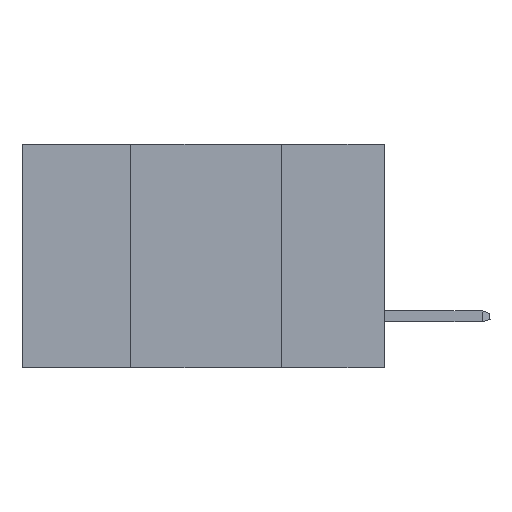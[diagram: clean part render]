
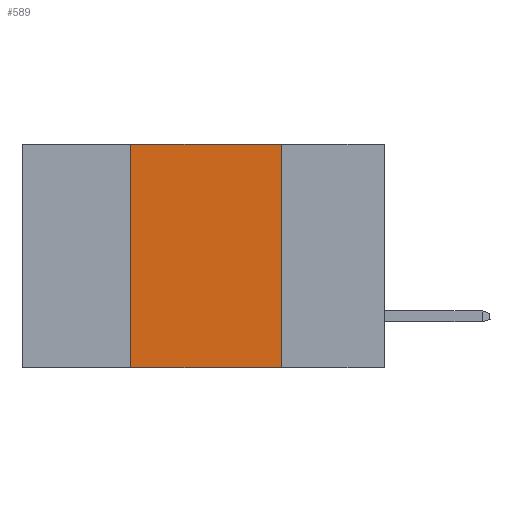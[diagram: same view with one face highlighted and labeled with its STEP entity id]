
A CAD part, left-side view. The second image highlights one B-rep face of the part: STEP entity #589.
In plain terms, the highlighted planar face has unit normal (-1, 0, 0).
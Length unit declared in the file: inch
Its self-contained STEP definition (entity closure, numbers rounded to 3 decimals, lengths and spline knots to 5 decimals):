
#203 = DIRECTION ( 'NONE',  ( 0., -1., 0. ) ) ;
#589 = ADVANCED_FACE ( 'NONE', ( #673 ), #17092, .F. ) ;
#673 = FACE_OUTER_BOUND ( 'NONE', #18029, .T. ) ;
#727 = ORIENTED_EDGE ( 'NONE', *, *, #7340, .T. ) ;
#878 = DIRECTION ( 'NONE',  ( 0., 0., -1. ) ) ;
#1044 = LINE ( 'NONE', #25369, #7837 ) ;
#1228 = VECTOR ( 'NONE', #203, 39.37008 ) ;
#3709 = EDGE_CURVE ( 'NONE', #28341, #19710, #4399, .T. ) ;
#4399 = LINE ( 'NONE', #16062, #1228 ) ;
#4417 = CARTESIAN_POINT ( 'NONE',  ( 0., 0.17, 0. ) ) ;
#4622 = ORIENTED_EDGE ( 'NONE', *, *, #18394, .F. ) ;
#5291 = ORIENTED_EDGE ( 'NONE', *, *, #9545, .F. ) ;
#7340 = EDGE_CURVE ( 'NONE', #24882, #21095, #1044, .T. ) ;
#7837 = VECTOR ( 'NONE', #13984, 39.37008 ) ;
#8672 = CARTESIAN_POINT ( 'NONE',  ( 0., 0.17, 0. ) ) ;
#9545 = EDGE_CURVE ( 'NONE', #19710, #21095, #14792, .T. ) ;
#11302 = CARTESIAN_POINT ( 'NONE',  ( 0., 0.42, 0. ) ) ;
#12245 = CARTESIAN_POINT ( 'NONE',  ( 0., 0.6, 0. ) ) ;
#12881 = AXIS2_PLACEMENT_3D ( 'NONE', #12245, #28190, #878 ) ;
#13799 = DIRECTION ( 'NONE',  ( 0., 0., 1. ) ) ;
#13984 = DIRECTION ( 'NONE',  ( 0., -1., 0. ) ) ;
#14336 = CARTESIAN_POINT ( 'NONE',  ( 0., 0.42, 0. ) ) ;
#14792 = LINE ( 'NONE', #8672, #24062 ) ;
#15138 = DIRECTION ( 'NONE',  ( 0., 0., -1. ) ) ;
#16062 = CARTESIAN_POINT ( 'NONE',  ( 0., 0.6, 0. ) ) ;
#17092 = PLANE ( 'NONE',  #12881 ) ;
#17466 = VECTOR ( 'NONE', #13799, 39.37008 ) ;
#17570 = CARTESIAN_POINT ( 'NONE',  ( 0., 0.17, -0.37 ) ) ;
#18029 = EDGE_LOOP ( 'NONE', ( #5291, #25654, #4622, #727 ) ) ;
#18394 = EDGE_CURVE ( 'NONE', #24882, #28341, #28878, .T. ) ;
#19710 = VERTEX_POINT ( 'NONE', #4417 ) ;
#20025 = CARTESIAN_POINT ( 'NONE',  ( 0., 0.42, -0.37 ) ) ;
#21095 = VERTEX_POINT ( 'NONE', #17570 ) ;
#24062 = VECTOR ( 'NONE', #15138, 39.37008 ) ;
#24882 = VERTEX_POINT ( 'NONE', #20025 ) ;
#25369 = CARTESIAN_POINT ( 'NONE',  ( 0., 0.6, -0.37 ) ) ;
#25654 = ORIENTED_EDGE ( 'NONE', *, *, #3709, .F. ) ;
#28190 = DIRECTION ( 'NONE',  ( 1., 0., 0. ) ) ;
#28341 = VERTEX_POINT ( 'NONE', #14336 ) ;
#28878 = LINE ( 'NONE', #11302, #17466 ) ;
